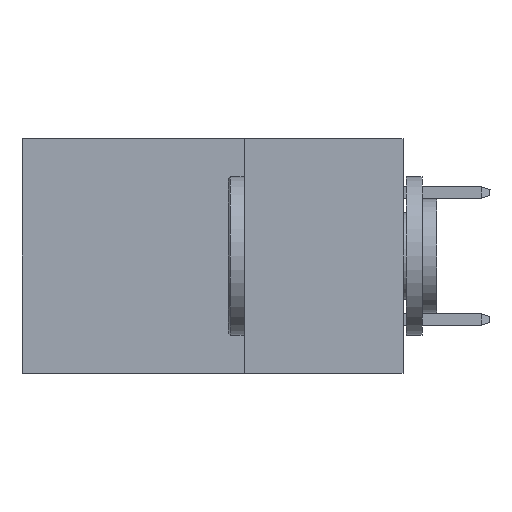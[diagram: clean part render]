
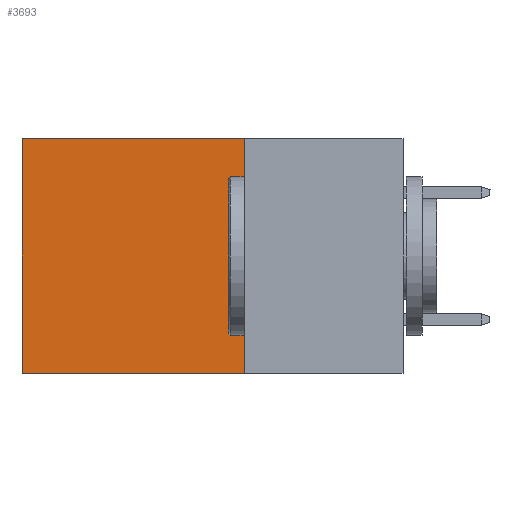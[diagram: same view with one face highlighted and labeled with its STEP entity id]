
A CAD part, left-side view. The second image highlights one B-rep face of the part: STEP entity #3693.
In plain terms, the highlighted planar face has unit normal (-1, 0, 0).
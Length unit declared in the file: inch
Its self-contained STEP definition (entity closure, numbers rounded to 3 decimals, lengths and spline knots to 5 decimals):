
#189 = CARTESIAN_POINT ( 'NONE',  ( 0.2875, 0.25, -0.37 ) ) ;
#300 = CARTESIAN_POINT ( 'NONE',  ( 0.2875, 0.6, -0.37 ) ) ;
#942 = CARTESIAN_POINT ( 'NONE',  ( 0.2875, 0.6, 0. ) ) ;
#1234 = CARTESIAN_POINT ( 'NONE',  ( 0.2875, 0.25, -0.37 ) ) ;
#1463 = VECTOR ( 'NONE', #23275, 39.37008 ) ;
#1627 = DIRECTION ( 'NONE',  ( 0., 0., -1. ) ) ;
#2471 = LINE ( 'NONE', #189, #1463 ) ;
#3693 = ADVANCED_FACE ( 'NONE', ( #22586 ), #4035, .F. ) ;
#4035 = PLANE ( 'NONE',  #28178 ) ;
#5720 = CARTESIAN_POINT ( 'NONE',  ( 0.2875, 0.25, 0. ) ) ;
#6447 = DIRECTION ( 'NONE',  ( 1., 0., 0. ) ) ;
#6840 = EDGE_CURVE ( 'NONE', #20894, #9058, #17460, .T. ) ;
#6897 = DIRECTION ( 'NONE',  ( 0., 1., 0. ) ) ;
#9058 = VERTEX_POINT ( 'NONE', #1234 ) ;
#10196 = EDGE_CURVE ( 'NONE', #9058, #20018, #2471, .T. ) ;
#10320 = EDGE_CURVE ( 'NONE', #26146, #20018, #17365, .T. ) ;
#11293 = VECTOR ( 'NONE', #28639, 39.37008 ) ;
#13830 = CARTESIAN_POINT ( 'NONE',  ( 0.2875, 0.25, 0. ) ) ;
#17048 = ORIENTED_EDGE ( 'NONE', *, *, #10320, .T. ) ;
#17276 = ORIENTED_EDGE ( 'NONE', *, *, #6840, .F. ) ;
#17365 = LINE ( 'NONE', #942, #18310 ) ;
#17460 = LINE ( 'NONE', #5720, #11293 ) ;
#18310 = VECTOR ( 'NONE', #19781, 39.37008 ) ;
#18934 = LINE ( 'NONE', #13830, #29174 ) ;
#19109 = ORIENTED_EDGE ( 'NONE', *, *, #10196, .F. ) ;
#19781 = DIRECTION ( 'NONE',  ( 0., 0., -1. ) ) ;
#20018 = VERTEX_POINT ( 'NONE', #300 ) ;
#20466 = CARTESIAN_POINT ( 'NONE',  ( 0.2875, 0.25, 0. ) ) ;
#20894 = VERTEX_POINT ( 'NONE', #24399 ) ;
#22438 = EDGE_CURVE ( 'NONE', #20894, #26146, #18934, .T. ) ;
#22586 = FACE_OUTER_BOUND ( 'NONE', #22814, .T. ) ;
#22814 = EDGE_LOOP ( 'NONE', ( #17048, #19109, #17276, #26296 ) ) ;
#23275 = DIRECTION ( 'NONE',  ( 0., 1., 0. ) ) ;
#24399 = CARTESIAN_POINT ( 'NONE',  ( 0.2875, 0.25, 0. ) ) ;
#26146 = VERTEX_POINT ( 'NONE', #28181 ) ;
#26296 = ORIENTED_EDGE ( 'NONE', *, *, #22438, .T. ) ;
#28178 = AXIS2_PLACEMENT_3D ( 'NONE', #20466, #6447, #1627 ) ;
#28181 = CARTESIAN_POINT ( 'NONE',  ( 0.2875, 0.6, 0. ) ) ;
#28639 = DIRECTION ( 'NONE',  ( 0., 0., -1. ) ) ;
#29174 = VECTOR ( 'NONE', #6897, 39.37008 ) ;
